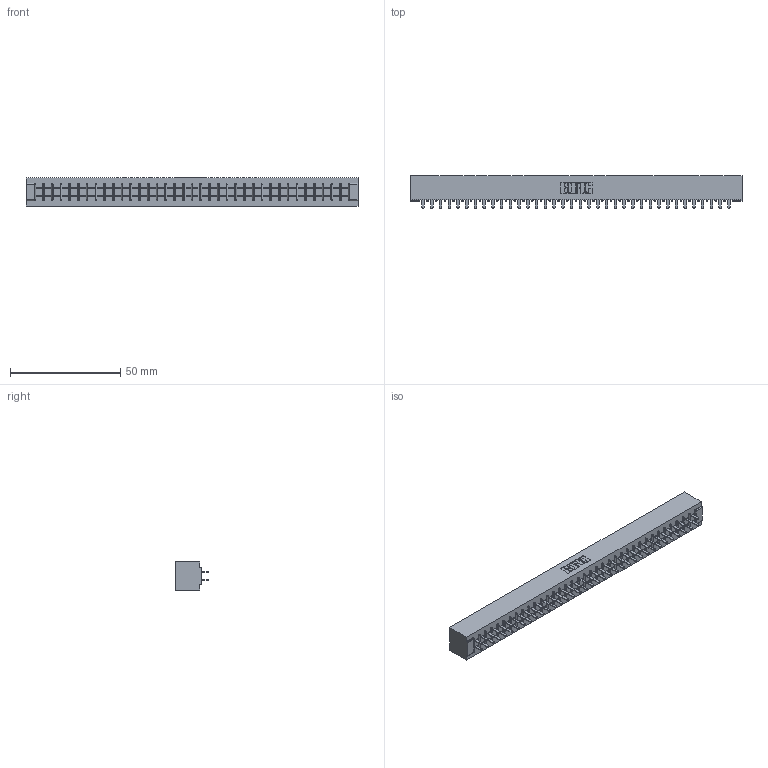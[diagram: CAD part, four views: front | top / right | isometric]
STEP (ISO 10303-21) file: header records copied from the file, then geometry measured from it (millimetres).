
FILE_DESCRIPTION (( 'STEP AP203' ), '1' );
FILE_NAME ('355-072-521-201.STEP', '2019-09-13T12:06:34', ( '' ), ( '' ), 'SwSTEP 2.0', 'SolidWorks 2016', '' );
FILE_SCHEMA (( 'CONFIG_CONTROL_DESIGN' ));
Length unit declared in the file: inch
Products named in the file (3): 355-072-521-201; 305-290-001_521; 305 Part_No Mounting
Assembly tree (73 placements, depth 2):
  355-072-521-201
    305 Part_No Mounting
    305-290-001_521  x72
Bounding box: 150.52 x 14.86 x 12.7 mm (x, y, z)
Volume: 16079.4 mm3; surface area: 20394.5 mm2
Topology: 73 solids, 73 shells, 3420 faces, 9760 edges, 6312 vertices
Faces by surface type: plane 2008, cylinder 1268, sphere 144
Entity records: 39311 total; most frequent: CARTESIAN_POINT 6502, ORIENTED_EDGE 6452, DIRECTION 6292, EDGE_CURVE 3226, VECTOR 2608, LINE 2608, VERTEX_POINT 2052, AXIS2_PLACEMENT_3D 1842
